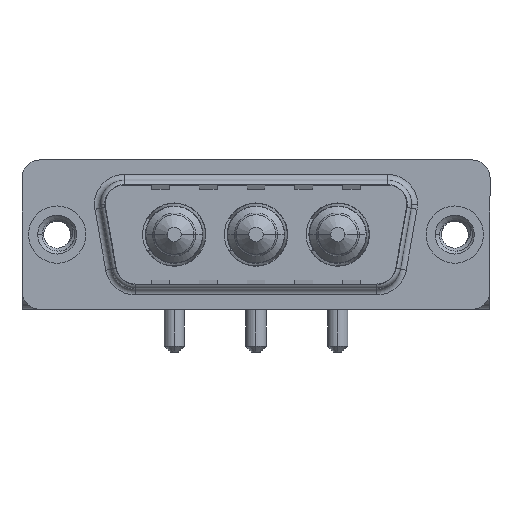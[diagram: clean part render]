
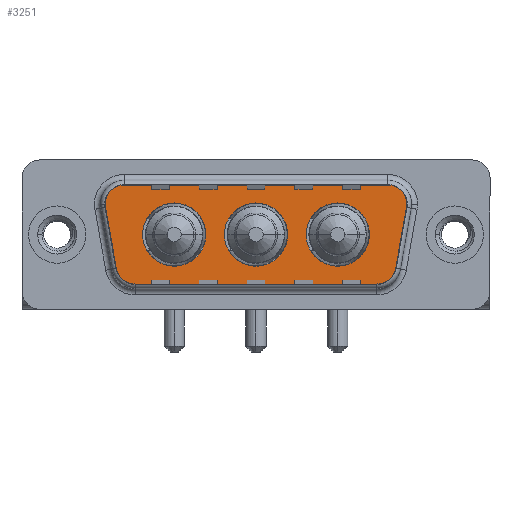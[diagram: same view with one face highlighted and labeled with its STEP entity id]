
A CAD part, top view. The second image highlights one B-rep face of the part: STEP entity #3251.
In plain terms, the highlighted planar face has unit normal (0, 0, 1).
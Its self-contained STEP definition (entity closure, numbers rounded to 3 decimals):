
#7 = EDGE_CURVE ( 'NONE', #9392, #10520, #7306, .T. ) ;
#14 = EDGE_CURVE ( 'NONE', #5575, #10012, #10834, .T. ) ;
#39 = DIRECTION ( 'NONE',  ( -1., 0., 0. ) ) ;
#219 = VERTEX_POINT ( 'NONE', #3956 ) ;
#287 = CARTESIAN_POINT ( 'NONE',  ( 3.441, 2.553, 0. ) ) ;
#374 = AXIS2_PLACEMENT_3D ( 'NONE', #12928, #8774, #11896 ) ;
#399 = AXIS2_PLACEMENT_3D ( 'NONE', #5129, #12594, #13541 ) ;
#503 = ORIENTED_EDGE ( 'NONE', *, *, #7374, .F. ) ;
#573 = CARTESIAN_POINT ( 'NONE',  ( 12.45, 0., 0. ) ) ;
#682 = DIRECTION ( 'NONE',  ( 0.174, -0.985, 0. ) ) ;
#819 = CIRCLE ( 'NONE', #8751, 2.65 ) ;
#896 = CARTESIAN_POINT ( 'NONE',  ( 5.411, 4.9, 0. ) ) ;
#913 = DIRECTION ( 'NONE',  ( 0.174, 0.985, 0. ) ) ;
#1011 = ORIENTED_EDGE ( 'NONE', *, *, #7, .T. ) ;
#1123 = CARTESIAN_POINT ( 'NONE',  ( 27.889, 4.9, 0. ) ) ;
#1133 = CARTESIAN_POINT ( 'NONE',  ( 23.5, 0., 0. ) ) ;
#1198 = DIRECTION ( 'NONE',  ( -1., 0., 0. ) ) ;
#1214 = DIRECTION ( 'NONE',  ( 0., 0., 1. ) ) ;
#1253 = CIRCLE ( 'NONE', #374, 2.65 ) ;
#1388 = ORIENTED_EDGE ( 'NONE', *, *, #5556, .F. ) ;
#1622 = LINE ( 'NONE', #6887, #4630 ) ;
#1637 = CIRCLE ( 'NONE', #9365, 2. ) ;
#1698 = ORIENTED_EDGE ( 'NONE', *, *, #4311, .T. ) ;
#1921 = FACE_BOUND ( 'NONE', #3781, .T. ) ;
#1934 = CIRCLE ( 'NONE', #2384, 2. ) ;
#1946 = EDGE_LOOP ( 'NONE', ( #7571, #10935 ) ) ;
#2172 = DIRECTION ( 'NONE',  ( 0., 0., 1. ) ) ;
#2187 = DIRECTION ( 'NONE',  ( 0., 0., 1. ) ) ;
#2204 = PLANE ( 'NONE',  #2740 ) ;
#2246 = VERTEX_POINT ( 'NONE', #3078 ) ;
#2266 = DIRECTION ( 'NONE',  ( 1., 0., 0. ) ) ;
#2311 = DIRECTION ( 'NONE',  ( 0., 0., 1. ) ) ;
#2384 = AXIS2_PLACEMENT_3D ( 'NONE', #7294, #4033, #39 ) ;
#2598 = DIRECTION ( 'NONE',  ( 0., 0., 1. ) ) ;
#2740 = AXIS2_PLACEMENT_3D ( 'NONE', #6490, #1214, #2266 ) ;
#2796 = CARTESIAN_POINT ( 'NONE',  ( 26.866, -4.9, 0. ) ) ;
#2831 = VERTEX_POINT ( 'NONE', #1123 ) ;
#2982 = CARTESIAN_POINT ( 'NONE',  ( 29.859, 2.553, 0. ) ) ;
#3078 = CARTESIAN_POINT ( 'NONE',  ( 6.434, -4.9, 0. ) ) ;
#3206 = DIRECTION ( 'NONE',  ( 0., 0., 1. ) ) ;
#3251 = ADVANCED_FACE ( 'NONE', ( #1921, #6149, #10359, #5104 ), #2204, .T. ) ;
#3295 = VERTEX_POINT ( 'NONE', #8553 ) ;
#3417 = CARTESIAN_POINT ( 'NONE',  ( 5.411, 2.9, 0. ) ) ;
#3687 = VECTOR ( 'NONE', #913, 1000. ) ;
#3744 = EDGE_CURVE ( 'NONE', #10429, #4075, #4612, .T. ) ;
#3781 = EDGE_LOOP ( 'NONE', ( #1388, #5282 ) ) ;
#3861 = DIRECTION ( 'NONE',  ( 0., 0., 1. ) ) ;
#3956 = CARTESIAN_POINT ( 'NONE',  ( 28.836, -3.247, 0. ) ) ;
#4033 = DIRECTION ( 'NONE',  ( 0., 0., 1. ) ) ;
#4075 = VERTEX_POINT ( 'NONE', #573 ) ;
#4191 = EDGE_CURVE ( 'NONE', #6301, #3295, #8649, .T. ) ;
#4257 = CARTESIAN_POINT ( 'NONE',  ( 9.8, 0., 0. ) ) ;
#4311 = EDGE_CURVE ( 'NONE', #10520, #7991, #7935, .T. ) ;
#4382 = DIRECTION ( 'NONE',  ( 1., 0., 0. ) ) ;
#4388 = ORIENTED_EDGE ( 'NONE', *, *, #6250, .T. ) ;
#4393 = DIRECTION ( 'NONE',  ( -1., 0., 0. ) ) ;
#4579 = CIRCLE ( 'NONE', #10518, 2. ) ;
#4612 = CIRCLE ( 'NONE', #12781, 2.65 ) ;
#4613 = VECTOR ( 'NONE', #4393, 1000. ) ;
#4630 = VECTOR ( 'NONE', #13098, 1000. ) ;
#4684 = ORIENTED_EDGE ( 'NONE', *, *, #9874, .T. ) ;
#4765 = VERTEX_POINT ( 'NONE', #10697 ) ;
#5104 = FACE_OUTER_BOUND ( 'NONE', #5776, .T. ) ;
#5129 = CARTESIAN_POINT ( 'NONE',  ( 9.8, 0., 0. ) ) ;
#5282 = ORIENTED_EDGE ( 'NONE', *, *, #4191, .F. ) ;
#5346 = CARTESIAN_POINT ( 'NONE',  ( 26.15, 0., 0. ) ) ;
#5475 = VERTEX_POINT ( 'NONE', #5346 ) ;
#5556 = EDGE_CURVE ( 'NONE', #3295, #6301, #1253, .T. ) ;
#5575 = VERTEX_POINT ( 'NONE', #11690 ) ;
#5776 = EDGE_LOOP ( 'NONE', ( #11889, #11819, #5980, #7909, #4684, #1011, #1698, #4388, #9103 ) ) ;
#5794 = EDGE_CURVE ( 'NONE', #10727, #219, #4579, .T. ) ;
#5980 = ORIENTED_EDGE ( 'NONE', *, *, #14, .T. ) ;
#6149 = FACE_BOUND ( 'NONE', #13069, .T. ) ;
#6250 = EDGE_CURVE ( 'NONE', #7991, #2246, #1637, .T. ) ;
#6301 = VERTEX_POINT ( 'NONE', #13440 ) ;
#6480 = DIRECTION ( 'NONE',  ( 0., 0., 1. ) ) ;
#6490 = CARTESIAN_POINT ( 'NONE',  ( 26.866, -2.9, 0. ) ) ;
#6651 = DIRECTION ( 'NONE',  ( 0., 0., 1. ) ) ;
#6887 = CARTESIAN_POINT ( 'NONE',  ( 6.434, -4.9, 0. ) ) ;
#7294 = CARTESIAN_POINT ( 'NONE',  ( 27.889, 2.9, 0. ) ) ;
#7306 = CIRCLE ( 'NONE', #11939, 2. ) ;
#7374 = EDGE_CURVE ( 'NONE', #4765, #5475, #12941, .T. ) ;
#7571 = ORIENTED_EDGE ( 'NONE', *, *, #11403, .F. ) ;
#7782 = DIRECTION ( 'NONE',  ( -1., 0., 0. ) ) ;
#7834 = ORIENTED_EDGE ( 'NONE', *, *, #8443, .F. ) ;
#7909 = ORIENTED_EDGE ( 'NONE', *, *, #10917, .T. ) ;
#7935 = LINE ( 'NONE', #13247, #9353 ) ;
#7991 = VERTEX_POINT ( 'NONE', #10476 ) ;
#8079 = AXIS2_PLACEMENT_3D ( 'NONE', #13329, #3861, #11330 ) ;
#8302 = LINE ( 'NONE', #2982, #3687 ) ;
#8346 = CIRCLE ( 'NONE', #399, 2.65 ) ;
#8443 = EDGE_CURVE ( 'NONE', #5475, #4765, #819, .T. ) ;
#8454 = DIRECTION ( 'NONE',  ( 1., 0., 0. ) ) ;
#8553 = CARTESIAN_POINT ( 'NONE',  ( 19.3, 0., 0. ) ) ;
#8649 = CIRCLE ( 'NONE', #10637, 2.65 ) ;
#8751 = AXIS2_PLACEMENT_3D ( 'NONE', #1133, #3206, #8454 ) ;
#8774 = DIRECTION ( 'NONE',  ( 0., 0., 1. ) ) ;
#8909 = CARTESIAN_POINT ( 'NONE',  ( 29.889, 2.9, 0. ) ) ;
#9045 = AXIS2_PLACEMENT_3D ( 'NONE', #10673, #2187, #1198 ) ;
#9103 = ORIENTED_EDGE ( 'NONE', *, *, #9711, .T. ) ;
#9353 = VECTOR ( 'NONE', #682, 1000. ) ;
#9365 = AXIS2_PLACEMENT_3D ( 'NONE', #11875, #2598, #7782 ) ;
#9392 = VERTEX_POINT ( 'NONE', #896 ) ;
#9482 = CARTESIAN_POINT ( 'NONE',  ( 16.65, 0., 0. ) ) ;
#9630 = LINE ( 'NONE', #10534, #4613 ) ;
#9711 = EDGE_CURVE ( 'NONE', #2246, #10727, #1622, .T. ) ;
#9874 = EDGE_CURVE ( 'NONE', #2831, #9392, #9630, .T. ) ;
#10012 = VERTEX_POINT ( 'NONE', #8909 ) ;
#10359 = FACE_BOUND ( 'NONE', #1946, .T. ) ;
#10429 = VERTEX_POINT ( 'NONE', #10790 ) ;
#10476 = CARTESIAN_POINT ( 'NONE',  ( 4.464, -3.247, 0. ) ) ;
#10518 = AXIS2_PLACEMENT_3D ( 'NONE', #12993, #6651, #10901 ) ;
#10520 = VERTEX_POINT ( 'NONE', #287 ) ;
#10534 = CARTESIAN_POINT ( 'NONE',  ( 5.411, 4.9, 0. ) ) ;
#10611 = DIRECTION ( 'NONE',  ( 1., 0., 0. ) ) ;
#10637 = AXIS2_PLACEMENT_3D ( 'NONE', #9482, #2172, #4382 ) ;
#10673 = CARTESIAN_POINT ( 'NONE',  ( 27.889, 2.9, 0. ) ) ;
#10676 = DIRECTION ( 'NONE',  ( 1., 0., 0. ) ) ;
#10697 = CARTESIAN_POINT ( 'NONE',  ( 20.85, 0., 0. ) ) ;
#10727 = VERTEX_POINT ( 'NONE', #2796 ) ;
#10790 = CARTESIAN_POINT ( 'NONE',  ( 7.15, 0., 0. ) ) ;
#10834 = CIRCLE ( 'NONE', #9045, 2. ) ;
#10901 = DIRECTION ( 'NONE',  ( 1., 0., 0. ) ) ;
#10917 = EDGE_CURVE ( 'NONE', #10012, #2831, #1934, .T. ) ;
#10935 = ORIENTED_EDGE ( 'NONE', *, *, #3744, .F. ) ;
#11330 = DIRECTION ( 'NONE',  ( 1., 0., 0. ) ) ;
#11401 = EDGE_CURVE ( 'NONE', #219, #5575, #8302, .T. ) ;
#11403 = EDGE_CURVE ( 'NONE', #4075, #10429, #8346, .T. ) ;
#11690 = CARTESIAN_POINT ( 'NONE',  ( 29.859, 2.553, 0. ) ) ;
#11819 = ORIENTED_EDGE ( 'NONE', *, *, #11401, .T. ) ;
#11875 = CARTESIAN_POINT ( 'NONE',  ( 6.434, -2.9, 0. ) ) ;
#11889 = ORIENTED_EDGE ( 'NONE', *, *, #5794, .T. ) ;
#11896 = DIRECTION ( 'NONE',  ( 1., 0., 0. ) ) ;
#11939 = AXIS2_PLACEMENT_3D ( 'NONE', #3417, #2311, #10611 ) ;
#12594 = DIRECTION ( 'NONE',  ( 0., 0., 1. ) ) ;
#12781 = AXIS2_PLACEMENT_3D ( 'NONE', #4257, #6480, #10676 ) ;
#12928 = CARTESIAN_POINT ( 'NONE',  ( 16.65, 0., 0. ) ) ;
#12941 = CIRCLE ( 'NONE', #8079, 2.65 ) ;
#12993 = CARTESIAN_POINT ( 'NONE',  ( 26.866, -2.9, 0. ) ) ;
#13069 = EDGE_LOOP ( 'NONE', ( #7834, #503 ) ) ;
#13098 = DIRECTION ( 'NONE',  ( 1., 0., 0. ) ) ;
#13247 = CARTESIAN_POINT ( 'NONE',  ( 3.441, 2.553, 0. ) ) ;
#13329 = CARTESIAN_POINT ( 'NONE',  ( 23.5, 0., 0. ) ) ;
#13440 = CARTESIAN_POINT ( 'NONE',  ( 14., 0., 0. ) ) ;
#13541 = DIRECTION ( 'NONE',  ( 1., 0., 0. ) ) ;
